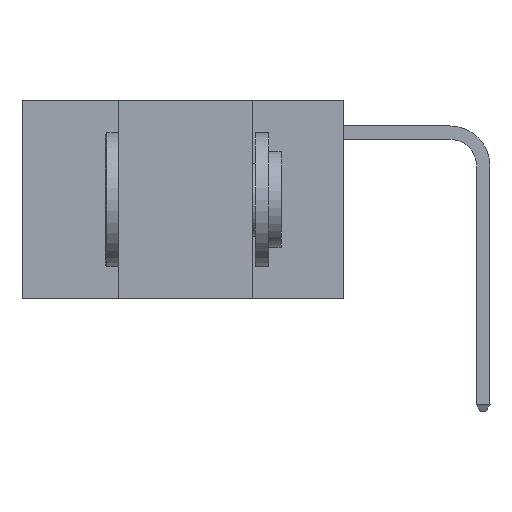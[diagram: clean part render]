
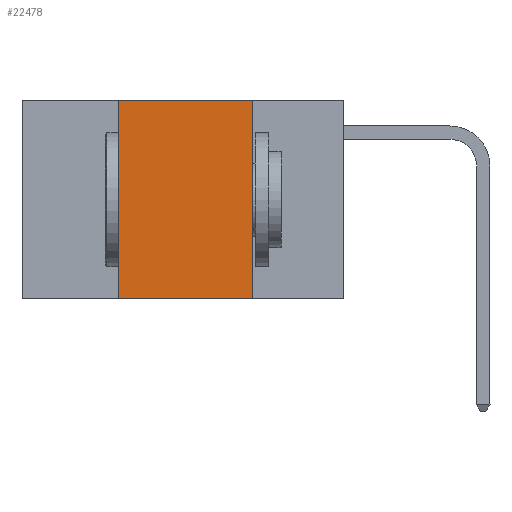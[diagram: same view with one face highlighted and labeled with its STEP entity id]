
A CAD part, left-side view. The second image highlights one B-rep face of the part: STEP entity #22478.
In plain terms, the highlighted planar face has unit normal (-1, 0, 0).
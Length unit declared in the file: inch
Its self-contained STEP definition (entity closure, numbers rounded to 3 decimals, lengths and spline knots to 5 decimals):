
#568 = DIRECTION ( 'NONE',  ( 0., -1., 0. ) ) ;
#729 = ORIENTED_EDGE ( 'NONE', *, *, #3325, .T. ) ;
#1246 = PLANE ( 'NONE',  #22141 ) ;
#1579 = DIRECTION ( 'NONE',  ( 1., 0., 0. ) ) ;
#1733 = VECTOR ( 'NONE', #568, 39.37008 ) ;
#1862 = EDGE_CURVE ( 'NONE', #5466, #14021, #4477, .T. ) ;
#2408 = VECTOR ( 'NONE', #2699, 39.37008 ) ;
#2444 = VECTOR ( 'NONE', #13727, 39.37008 ) ;
#2586 = LINE ( 'NONE', #11190, #2408 ) ;
#2699 = DIRECTION ( 'NONE',  ( 0., 0., 1. ) ) ;
#2865 = CARTESIAN_POINT ( 'NONE',  ( 0., 0.42, -0.37 ) ) ;
#3318 = CARTESIAN_POINT ( 'NONE',  ( 0., 0.6, 0. ) ) ;
#3325 = EDGE_CURVE ( 'NONE', #22272, #14021, #19728, .T. ) ;
#3383 = CARTESIAN_POINT ( 'NONE',  ( 0., 0.6, 0. ) ) ;
#4477 = LINE ( 'NONE', #18608, #6972 ) ;
#5466 = VERTEX_POINT ( 'NONE', #16567 ) ;
#5858 = ORIENTED_EDGE ( 'NONE', *, *, #1862, .F. ) ;
#6972 = VECTOR ( 'NONE', #10027, 39.37008 ) ;
#8308 = DIRECTION ( 'NONE',  ( 0., 0., -1. ) ) ;
#8791 = ORIENTED_EDGE ( 'NONE', *, *, #21458, .F. ) ;
#9290 = EDGE_LOOP ( 'NONE', ( #5858, #8791, #10282, #729 ) ) ;
#10027 = DIRECTION ( 'NONE',  ( 0., 0., -1. ) ) ;
#10282 = ORIENTED_EDGE ( 'NONE', *, *, #20194, .F. ) ;
#11190 = CARTESIAN_POINT ( 'NONE',  ( 0., 0.42, 0. ) ) ;
#11694 = CARTESIAN_POINT ( 'NONE',  ( 0., 0.42, 0. ) ) ;
#13727 = DIRECTION ( 'NONE',  ( 0., -1., 0. ) ) ;
#14021 = VERTEX_POINT ( 'NONE', #21546 ) ;
#16469 = CARTESIAN_POINT ( 'NONE',  ( 0., 0.6, -0.37 ) ) ;
#16567 = CARTESIAN_POINT ( 'NONE',  ( 0., 0.17, 0. ) ) ;
#17314 = LINE ( 'NONE', #3383, #2444 ) ;
#17474 = FACE_OUTER_BOUND ( 'NONE', #9290, .T. ) ;
#18608 = CARTESIAN_POINT ( 'NONE',  ( 0., 0.17, 0. ) ) ;
#19728 = LINE ( 'NONE', #16469, #1733 ) ;
#20194 = EDGE_CURVE ( 'NONE', #22272, #22229, #2586, .T. ) ;
#21458 = EDGE_CURVE ( 'NONE', #22229, #5466, #17314, .T. ) ;
#21546 = CARTESIAN_POINT ( 'NONE',  ( 0., 0.17, -0.37 ) ) ;
#22141 = AXIS2_PLACEMENT_3D ( 'NONE', #3318, #1579, #8308 ) ;
#22229 = VERTEX_POINT ( 'NONE', #11694 ) ;
#22272 = VERTEX_POINT ( 'NONE', #2865 ) ;
#22478 = ADVANCED_FACE ( 'NONE', ( #17474 ), #1246, .F. ) ;
